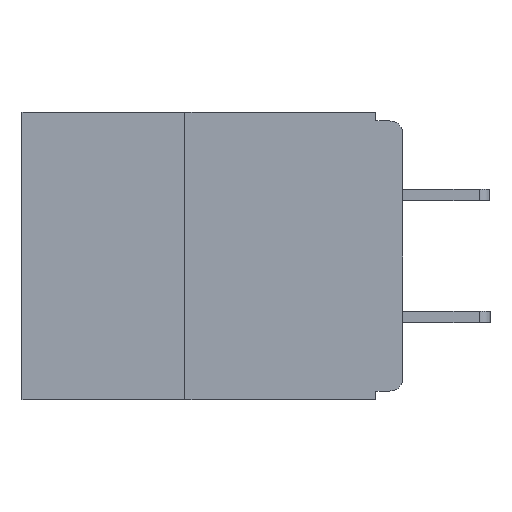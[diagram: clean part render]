
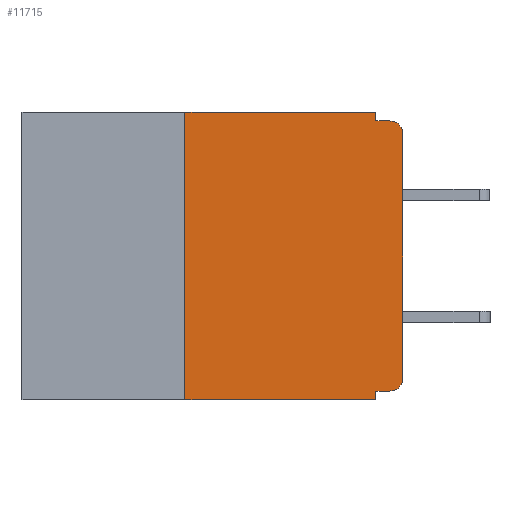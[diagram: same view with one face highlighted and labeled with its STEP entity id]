
A CAD part, left-side view. The second image highlights one B-rep face of the part: STEP entity #11715.
In plain terms, the highlighted planar face has unit normal (-1, 0, 0).
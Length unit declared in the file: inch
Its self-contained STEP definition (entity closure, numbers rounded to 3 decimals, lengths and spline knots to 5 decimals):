
#544 = CIRCLE ( 'NONE', #12335, 0.015 ) ;
#1551 = AXIS2_PLACEMENT_3D ( 'NONE', #24459, #11823, #26488 ) ;
#1946 = LINE ( 'NONE', #19348, #23087 ) ;
#2320 = VECTOR ( 'NONE', #4413, 39.37008 ) ;
#2395 = CARTESIAN_POINT ( 'NONE',  ( 0., 0.031, 0. ) ) ;
#2449 = VERTEX_POINT ( 'NONE', #6070 ) ;
#2671 = CARTESIAN_POINT ( 'NONE',  ( 0., 0.25, -0.33 ) ) ;
#3157 = EDGE_CURVE ( 'NONE', #14127, #2449, #26679, .T. ) ;
#3755 = VECTOR ( 'NONE', #21477, 39.37008 ) ;
#4413 = DIRECTION ( 'NONE',  ( 0., -1., 0. ) ) ;
#4573 = EDGE_CURVE ( 'NONE', #20742, #2449, #19852, .T. ) ;
#4801 = DIRECTION ( 'NONE',  ( 0., 0., 1. ) ) ;
#4823 = DIRECTION ( 'NONE',  ( 1., 0., 0. ) ) ;
#5199 = LINE ( 'NONE', #2671, #21414 ) ;
#5273 = EDGE_CURVE ( 'NONE', #15578, #12266, #1946, .T. ) ;
#5635 = CARTESIAN_POINT ( 'NONE',  ( 0., 0., 0. ) ) ;
#5953 = DIRECTION ( 'NONE',  ( 0., -1., 0. ) ) ;
#5976 = EDGE_CURVE ( 'NONE', #20742, #15451, #5199, .T. ) ;
#6070 = CARTESIAN_POINT ( 'NONE',  ( 0., 0.031, -0.33 ) ) ;
#6103 = CARTESIAN_POINT ( 'NONE',  ( 0., 0.031, 0. ) ) ;
#6466 = CARTESIAN_POINT ( 'NONE',  ( 0., 0.015, -0.025 ) ) ;
#6488 = FACE_OUTER_BOUND ( 'NONE', #6522, .T. ) ;
#6522 = EDGE_LOOP ( 'NONE', ( #14358, #14877, #15142, #15168, #15446, #15491, #15679, #15986, #16658, #17048 ) ) ;
#6603 = CARTESIAN_POINT ( 'NONE',  ( 0., 0., -0.305 ) ) ;
#8595 = DIRECTION ( 'NONE',  ( 0., 0., -1. ) ) ;
#9867 = VECTOR ( 'NONE', #24947, 39.37008 ) ;
#10220 = CARTESIAN_POINT ( 'NONE',  ( 0., 0.25, 0. ) ) ;
#10221 = EDGE_CURVE ( 'NONE', #16869, #15578, #16864, .T. ) ;
#10349 = VECTOR ( 'NONE', #5953, 39.37008 ) ;
#11508 = AXIS2_PLACEMENT_3D ( 'NONE', #21630, #4823, #19611 ) ;
#11715 = ADVANCED_FACE ( 'NONE', ( #6488 ), #17502, .F. ) ;
#11823 = DIRECTION ( 'NONE',  ( -1., 0., 0. ) ) ;
#11833 = CARTESIAN_POINT ( 'NONE',  ( 0., 0.015, -0.32 ) ) ;
#12266 = VERTEX_POINT ( 'NONE', #19686 ) ;
#12335 = AXIS2_PLACEMENT_3D ( 'NONE', #6466, #21251, #8595 ) ;
#12754 = CARTESIAN_POINT ( 'NONE',  ( 0., 0.437, -0.33 ) ) ;
#12923 = LINE ( 'NONE', #5635, #13601 ) ;
#13601 = VECTOR ( 'NONE', #16206, 39.37008 ) ;
#13753 = EDGE_CURVE ( 'NONE', #22770, #14786, #12923, .T. ) ;
#14127 = VERTEX_POINT ( 'NONE', #21698 ) ;
#14358 = ORIENTED_EDGE ( 'NONE', *, *, #13753, .T. ) ;
#14786 = VERTEX_POINT ( 'NONE', #15199 ) ;
#14877 = ORIENTED_EDGE ( 'NONE', *, *, #19996, .T. ) ;
#14969 = LINE ( 'NONE', #19364, #3755 ) ;
#15142 = ORIENTED_EDGE ( 'NONE', *, *, #5273, .F. ) ;
#15146 = EDGE_CURVE ( 'NONE', #15451, #16869, #27009, .T. ) ;
#15165 = DIRECTION ( 'NONE',  ( 0., -1., 0. ) ) ;
#15168 = ORIENTED_EDGE ( 'NONE', *, *, #10221, .F. ) ;
#15199 = CARTESIAN_POINT ( 'NONE',  ( 0., 0., -0.025 ) ) ;
#15446 = ORIENTED_EDGE ( 'NONE', *, *, #15146, .F. ) ;
#15451 = VERTEX_POINT ( 'NONE', #10220 ) ;
#15469 = CARTESIAN_POINT ( 'NONE',  ( 0., 0.25, -0.33 ) ) ;
#15491 = ORIENTED_EDGE ( 'NONE', *, *, #5976, .F. ) ;
#15578 = VERTEX_POINT ( 'NONE', #21310 ) ;
#15679 = ORIENTED_EDGE ( 'NONE', *, *, #4573, .T. ) ;
#15909 = CIRCLE ( 'NONE', #1551, 0.015 ) ;
#15986 = ORIENTED_EDGE ( 'NONE', *, *, #3157, .F. ) ;
#16206 = DIRECTION ( 'NONE',  ( 0., 0., 1. ) ) ;
#16658 = ORIENTED_EDGE ( 'NONE', *, *, #22795, .F. ) ;
#16864 = LINE ( 'NONE', #6103, #9867 ) ;
#16869 = VERTEX_POINT ( 'NONE', #2395 ) ;
#17048 = ORIENTED_EDGE ( 'NONE', *, *, #17192, .T. ) ;
#17192 = EDGE_CURVE ( 'NONE', #20302, #22770, #15909, .T. ) ;
#17502 = PLANE ( 'NONE',  #11508 ) ;
#18153 = DIRECTION ( 'NONE',  ( 0., 0., -1. ) ) ;
#18250 = CARTESIAN_POINT ( 'NONE',  ( 0., 0.031, -0.33 ) ) ;
#18636 = CARTESIAN_POINT ( 'NONE',  ( 0., 0.437, 0. ) ) ;
#19348 = CARTESIAN_POINT ( 'NONE',  ( 0., 0., -0.01 ) ) ;
#19364 = CARTESIAN_POINT ( 'NONE',  ( 0., 0., -0.32 ) ) ;
#19611 = DIRECTION ( 'NONE',  ( 0., 0., -1. ) ) ;
#19686 = CARTESIAN_POINT ( 'NONE',  ( 0., 0.015, -0.01 ) ) ;
#19852 = LINE ( 'NONE', #12754, #2320 ) ;
#19996 = EDGE_CURVE ( 'NONE', #14786, #12266, #544, .T. ) ;
#20302 = VERTEX_POINT ( 'NONE', #11833 ) ;
#20742 = VERTEX_POINT ( 'NONE', #15469 ) ;
#21251 = DIRECTION ( 'NONE',  ( -1., 0., 0. ) ) ;
#21310 = CARTESIAN_POINT ( 'NONE',  ( 0., 0.031, -0.01 ) ) ;
#21414 = VECTOR ( 'NONE', #4801, 39.37008 ) ;
#21477 = DIRECTION ( 'NONE',  ( 0., 1., 0. ) ) ;
#21630 = CARTESIAN_POINT ( 'NONE',  ( 0., 0.437, 0. ) ) ;
#21698 = CARTESIAN_POINT ( 'NONE',  ( 0., 0.031, -0.32 ) ) ;
#21884 = VECTOR ( 'NONE', #18153, 39.37008 ) ;
#22770 = VERTEX_POINT ( 'NONE', #6603 ) ;
#22795 = EDGE_CURVE ( 'NONE', #20302, #14127, #14969, .T. ) ;
#23087 = VECTOR ( 'NONE', #15165, 39.37008 ) ;
#24459 = CARTESIAN_POINT ( 'NONE',  ( 0., 0.015, -0.305 ) ) ;
#24947 = DIRECTION ( 'NONE',  ( 0., 0., -1. ) ) ;
#26488 = DIRECTION ( 'NONE',  ( 0., 0., -1. ) ) ;
#26679 = LINE ( 'NONE', #18250, #21884 ) ;
#27009 = LINE ( 'NONE', #18636, #10349 ) ;
